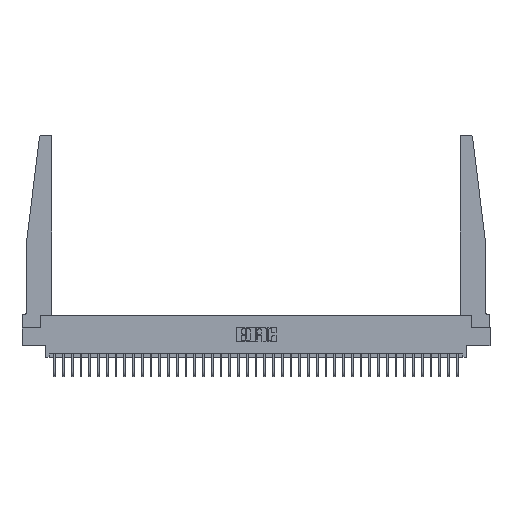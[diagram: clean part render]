
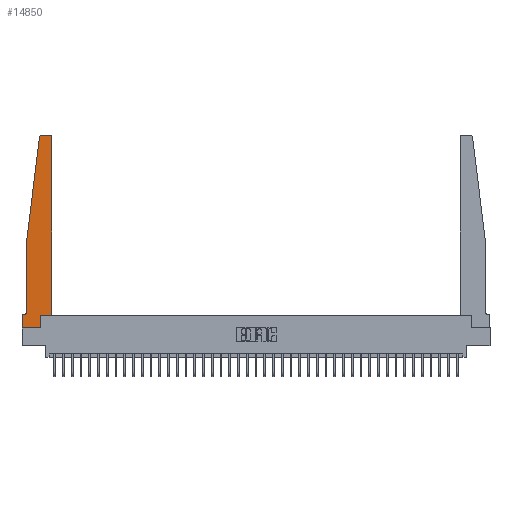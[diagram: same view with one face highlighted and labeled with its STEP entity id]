
A CAD part, top view. The second image highlights one B-rep face of the part: STEP entity #14850.
In plain terms, the highlighted planar face has unit normal (0, 0, 1).
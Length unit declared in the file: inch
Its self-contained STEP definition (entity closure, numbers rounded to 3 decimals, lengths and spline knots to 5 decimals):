
#68 = LINE ( 'NONE', #2313, #20347 ) ;
#532 = VECTOR ( 'NONE', #25959, 39.37008 ) ;
#581 = VECTOR ( 'NONE', #34279, 39.37008 ) ;
#615 = LINE ( 'NONE', #26376, #11274 ) ;
#653 = VERTEX_POINT ( 'NONE', #11686 ) ;
#1561 = CARTESIAN_POINT ( 'NONE',  ( 0.065, 1.25, 0.37 ) ) ;
#1821 = VECTOR ( 'NONE', #18164, 39.37008 ) ;
#2313 = CARTESIAN_POINT ( 'NONE',  ( 0.065, 1.25, 0.37 ) ) ;
#3034 = CARTESIAN_POINT ( 'NONE',  ( 0.395, 2.72, 0.37 ) ) ;
#3044 = ORIENTED_EDGE ( 'NONE', *, *, #14168, .T. ) ;
#3207 = CARTESIAN_POINT ( 'NONE',  ( 0.425, 2.72, 0.37 ) ) ;
#3563 = ORIENTED_EDGE ( 'NONE', *, *, #35480, .T. ) ;
#3842 = PLANE ( 'NONE',  #34864 ) ;
#4304 = ORIENTED_EDGE ( 'NONE', *, *, #13861, .T. ) ;
#4478 = DIRECTION ( 'NONE',  ( -1., 0., 0. ) ) ;
#5088 = CARTESIAN_POINT ( 'NONE',  ( 0.425, 0.18, 0.37 ) ) ;
#5094 = EDGE_CURVE ( 'NONE', #27888, #21035, #615, .T. ) ;
#5685 = DIRECTION ( 'NONE',  ( -1., 0., 0. ) ) ;
#5713 = EDGE_CURVE ( 'NONE', #19251, #23113, #68, .T. ) ;
#6168 = CARTESIAN_POINT ( 'NONE',  ( 0.27653, 2.72, 0.37 ) ) ;
#6407 = DIRECTION ( 'NONE',  ( 0., 0., 1. ) ) ;
#6692 = CARTESIAN_POINT ( 'NONE',  ( 0.425, 0.18, 0.37 ) ) ;
#6730 = CARTESIAN_POINT ( 'NONE',  ( 0.2605, 0., 0.37 ) ) ;
#7866 = CIRCLE ( 'NONE', #10276, 0.03 ) ;
#8105 = LINE ( 'NONE', #11666, #532 ) ;
#8227 = CARTESIAN_POINT ( 'NONE',  ( 0.065, 1.25, 0.37 ) ) ;
#8954 = AXIS2_PLACEMENT_3D ( 'NONE', #6168, #35495, #26845 ) ;
#9450 = VECTOR ( 'NONE', #17140, 39.37008 ) ;
#9995 = EDGE_CURVE ( 'NONE', #15420, #35702, #8105, .T. ) ;
#10059 = ORIENTED_EDGE ( 'NONE', *, *, #32852, .T. ) ;
#10276 = AXIS2_PLACEMENT_3D ( 'NONE', #3034, #6407, #31611 ) ;
#10732 = LINE ( 'NONE', #28419, #9450 ) ;
#11008 = EDGE_CURVE ( 'NONE', #36340, #20431, #16994, .T. ) ;
#11259 = VERTEX_POINT ( 'NONE', #24655 ) ;
#11274 = VECTOR ( 'NONE', #20365, 39.37008 ) ;
#11320 = LINE ( 'NONE', #13771, #25022 ) ;
#11518 = ORIENTED_EDGE ( 'NONE', *, *, #5094, .T. ) ;
#11666 = CARTESIAN_POINT ( 'NONE',  ( 0.425, 0.18, 0.37 ) ) ;
#11686 = CARTESIAN_POINT ( 'NONE',  ( 0., 0., 0.37 ) ) ;
#12023 = EDGE_CURVE ( 'NONE', #21035, #19251, #26383, .T. ) ;
#13743 = LINE ( 'NONE', #33867, #25089 ) ;
#13771 = CARTESIAN_POINT ( 'NONE',  ( 0.065, 0.1875, 0.37 ) ) ;
#13861 = EDGE_CURVE ( 'NONE', #18734, #31004, #15406, .T. ) ;
#14168 = EDGE_CURVE ( 'NONE', #23113, #18734, #17263, .T. ) ;
#14850 = ADVANCED_FACE ( 'NONE', ( #29610 ), #3842, .T. ) ;
#15319 = CARTESIAN_POINT ( 'NONE',  ( 0., 0.1875, 0.37 ) ) ;
#15406 = CIRCLE ( 'NONE', #21420, 0.05 ) ;
#15420 = VERTEX_POINT ( 'NONE', #5088 ) ;
#16508 = DIRECTION ( 'NONE',  ( 0., 0., -1. ) ) ;
#16994 = LINE ( 'NONE', #26379, #581 ) ;
#17140 = DIRECTION ( 'NONE',  ( 0., -1., 0. ) ) ;
#17263 = LINE ( 'NONE', #8227, #22596 ) ;
#18164 = DIRECTION ( 'NONE',  ( 1., 0., 0. ) ) ;
#18485 = CARTESIAN_POINT ( 'NONE',  ( 0.24675, 2.72367, 0.37 ) ) ;
#18734 = VERTEX_POINT ( 'NONE', #34715 ) ;
#19251 = VERTEX_POINT ( 'NONE', #18485 ) ;
#19704 = CARTESIAN_POINT ( 'NONE',  ( 0.015, 0.1875, 0.37 ) ) ;
#20347 = VECTOR ( 'NONE', #25831, 39.37008 ) ;
#20365 = DIRECTION ( 'NONE',  ( -1., 0., 0. ) ) ;
#20431 = VERTEX_POINT ( 'NONE', #27509 ) ;
#21035 = VERTEX_POINT ( 'NONE', #28210 ) ;
#21420 = AXIS2_PLACEMENT_3D ( 'NONE', #33615, #16508, #4478 ) ;
#21762 = ORIENTED_EDGE ( 'NONE', *, *, #11008, .T. ) ;
#22596 = VECTOR ( 'NONE', #34169, 39.37008 ) ;
#23113 = VERTEX_POINT ( 'NONE', #1561 ) ;
#23630 = LINE ( 'NONE', #6692, #1821 ) ;
#24655 = CARTESIAN_POINT ( 'NONE',  ( 0., 0.1875, 0.37 ) ) ;
#24910 = ORIENTED_EDGE ( 'NONE', *, *, #9995, .T. ) ;
#25022 = VECTOR ( 'NONE', #5685, 39.37008 ) ;
#25053 = CARTESIAN_POINT ( 'NONE',  ( 0.395, 2.75, 0.37 ) ) ;
#25089 = VECTOR ( 'NONE', #36132, 39.37008 ) ;
#25831 = DIRECTION ( 'NONE',  ( -0.122, -0.992, 0. ) ) ;
#25896 = ORIENTED_EDGE ( 'NONE', *, *, #33597, .T. ) ;
#25959 = DIRECTION ( 'NONE',  ( 0., 1., 0. ) ) ;
#26232 = EDGE_CURVE ( 'NONE', #31004, #11259, #11320, .T. ) ;
#26376 = CARTESIAN_POINT ( 'NONE',  ( 0.25, 2.75, 0.37 ) ) ;
#26379 = CARTESIAN_POINT ( 'NONE',  ( 0.2605, 0.18, 0.37 ) ) ;
#26383 = CIRCLE ( 'NONE', #8954, 0.03 ) ;
#26790 = DIRECTION ( 'NONE',  ( 0., 0., 1. ) ) ;
#26845 = DIRECTION ( 'NONE',  ( 1., 0., 0. ) ) ;
#26909 = ORIENTED_EDGE ( 'NONE', *, *, #12023, .T. ) ;
#27509 = CARTESIAN_POINT ( 'NONE',  ( 0.2605, 0.18, 0.37 ) ) ;
#27888 = VERTEX_POINT ( 'NONE', #25053 ) ;
#28210 = CARTESIAN_POINT ( 'NONE',  ( 0.27653, 2.75, 0.37 ) ) ;
#28419 = CARTESIAN_POINT ( 'NONE',  ( 0., 0., 0.37 ) ) ;
#29549 = EDGE_CURVE ( 'NONE', #653, #36340, #13743, .T. ) ;
#29610 = FACE_OUTER_BOUND ( 'NONE', #34339, .T. ) ;
#30763 = ORIENTED_EDGE ( 'NONE', *, *, #26232, .T. ) ;
#31004 = VERTEX_POINT ( 'NONE', #19704 ) ;
#31611 = DIRECTION ( 'NONE',  ( 1., 0., 0. ) ) ;
#32852 = EDGE_CURVE ( 'NONE', #20431, #15420, #23630, .T. ) ;
#33341 = DIRECTION ( 'NONE',  ( 1., 0., 0. ) ) ;
#33597 = EDGE_CURVE ( 'NONE', #35702, #27888, #7866, .T. ) ;
#33615 = CARTESIAN_POINT ( 'NONE',  ( 0.015, 0.2375, 0.37 ) ) ;
#33641 = ORIENTED_EDGE ( 'NONE', *, *, #5713, .T. ) ;
#33867 = CARTESIAN_POINT ( 'NONE',  ( 0., 0., 0.37 ) ) ;
#34169 = DIRECTION ( 'NONE',  ( 0., -1., 0. ) ) ;
#34194 = ORIENTED_EDGE ( 'NONE', *, *, #29549, .T. ) ;
#34279 = DIRECTION ( 'NONE',  ( 0., 1., 0. ) ) ;
#34339 = EDGE_LOOP ( 'NONE', ( #11518, #26909, #33641, #3044, #4304, #30763, #3563, #34194, #21762, #10059, #24910, #25896 ) ) ;
#34715 = CARTESIAN_POINT ( 'NONE',  ( 0.065, 0.2375, 0.37 ) ) ;
#34864 = AXIS2_PLACEMENT_3D ( 'NONE', #15319, #26790, #33341 ) ;
#35480 = EDGE_CURVE ( 'NONE', #11259, #653, #10732, .T. ) ;
#35495 = DIRECTION ( 'NONE',  ( 0., 0., 1. ) ) ;
#35702 = VERTEX_POINT ( 'NONE', #3207 ) ;
#36132 = DIRECTION ( 'NONE',  ( 1., 0., 0. ) ) ;
#36340 = VERTEX_POINT ( 'NONE', #6730 ) ;
